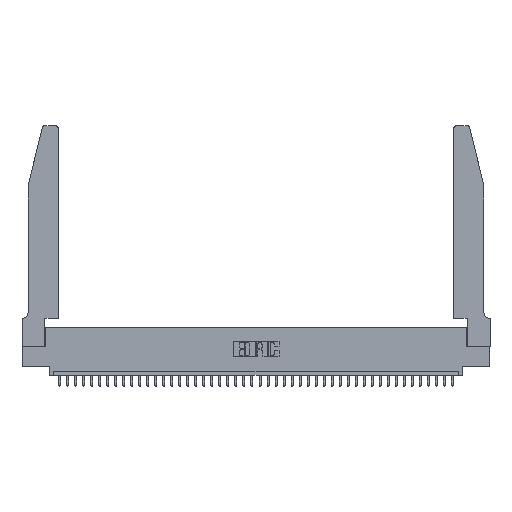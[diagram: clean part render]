
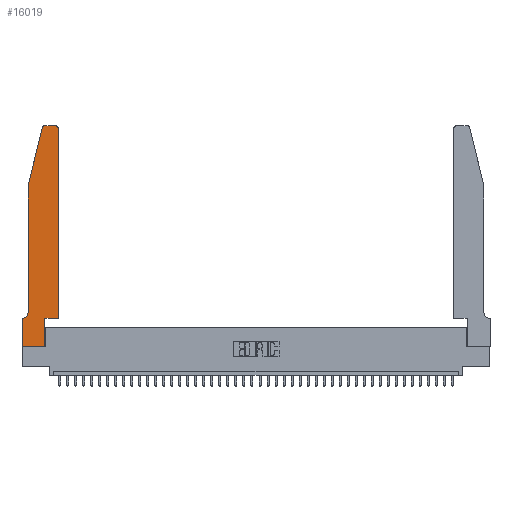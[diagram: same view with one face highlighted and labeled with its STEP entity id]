
A CAD part, top view. The second image highlights one B-rep face of the part: STEP entity #16019.
In plain terms, the highlighted planar face has unit normal (0, 0, 1).
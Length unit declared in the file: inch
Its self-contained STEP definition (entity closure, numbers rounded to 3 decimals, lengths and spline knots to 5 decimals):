
#346 = CARTESIAN_POINT ( 'NONE',  ( 0.25487, 2.72718, 0.37 ) ) ;
#736 = DIRECTION ( 'NONE',  ( -1., 0., 0. ) ) ;
#814 = EDGE_CURVE ( 'NONE', #9112, #20167, #5189, .T. ) ;
#1764 = AXIS2_PLACEMENT_3D ( 'NONE', #19782, #19914, #736 ) ;
#2838 = CARTESIAN_POINT ( 'NONE',  ( 0.4505, 0.35, 0.37 ) ) ;
#3013 = VERTEX_POINT ( 'NONE', #36718 ) ;
#3801 = ORIENTED_EDGE ( 'NONE', *, *, #39092, .T. ) ;
#3964 = ORIENTED_EDGE ( 'NONE', *, *, #16819, .T. ) ;
#4105 = CARTESIAN_POINT ( 'NONE',  ( 0., 0., 0.37 ) ) ;
#4216 = DIRECTION ( 'NONE',  ( 0., 1., 0. ) ) ;
#4330 = CARTESIAN_POINT ( 'NONE',  ( 0.4505, 0.35, 0.37 ) ) ;
#5189 = LINE ( 'NONE', #28190, #39154 ) ;
#5357 = DIRECTION ( 'NONE',  ( 1., 0., 0. ) ) ;
#5396 = VECTOR ( 'NONE', #35546, 39.37008 ) ;
#6058 = VERTEX_POINT ( 'NONE', #20160 ) ;
#6128 = ORIENTED_EDGE ( 'NONE', *, *, #37053, .T. ) ;
#6854 = ORIENTED_EDGE ( 'NONE', *, *, #814, .T. ) ;
#7038 = ORIENTED_EDGE ( 'NONE', *, *, #9373, .T. ) ;
#7457 = LINE ( 'NONE', #18163, #25952 ) ;
#8942 = LINE ( 'NONE', #23212, #30993 ) ;
#9038 = ORIENTED_EDGE ( 'NONE', *, *, #20512, .T. ) ;
#9095 = ORIENTED_EDGE ( 'NONE', *, *, #15731, .T. ) ;
#9112 = VERTEX_POINT ( 'NONE', #40099 ) ;
#9202 = CARTESIAN_POINT ( 'NONE',  ( 0., 0., 0.37 ) ) ;
#9373 = EDGE_CURVE ( 'NONE', #20611, #40476, #41179, .T. ) ;
#9575 = CARTESIAN_POINT ( 'NONE',  ( 0.0755, 0.35, 0.37 ) ) ;
#10657 = CARTESIAN_POINT ( 'NONE',  ( 0.4505, 0.35, 0.37 ) ) ;
#10990 = VECTOR ( 'NONE', #4216, 39.37008 ) ;
#11147 = ORIENTED_EDGE ( 'NONE', *, *, #37629, .T. ) ;
#11154 = VECTOR ( 'NONE', #32223, 39.37008 ) ;
#11833 = LINE ( 'NONE', #2838, #12321 ) ;
#12281 = VECTOR ( 'NONE', #18586, 39.37008 ) ;
#12321 = VECTOR ( 'NONE', #25205, 39.37008 ) ;
#12413 = DIRECTION ( 'NONE',  ( 1., 0., 0. ) ) ;
#12538 = AXIS2_PLACEMENT_3D ( 'NONE', #27901, #40463, #5357 ) ;
#12904 = EDGE_CURVE ( 'NONE', #3013, #34636, #13747, .T. ) ;
#13071 = VERTEX_POINT ( 'NONE', #23274 ) ;
#13747 = CIRCLE ( 'NONE', #12538, 0.03 ) ;
#14055 = EDGE_CURVE ( 'NONE', #18879, #13071, #20097, .T. ) ;
#14204 = AXIS2_PLACEMENT_3D ( 'NONE', #18815, #34764, #12413 ) ;
#15124 = CARTESIAN_POINT ( 'NONE',  ( 0.0755, 2., 0.37 ) ) ;
#15313 = DIRECTION ( 'NONE',  ( 0., -1., 0. ) ) ;
#15731 = EDGE_CURVE ( 'NONE', #34792, #18879, #19470, .T. ) ;
#16019 = ADVANCED_FACE ( 'NONE', ( #33484 ), #28220, .T. ) ;
#16699 = CARTESIAN_POINT ( 'NONE',  ( 0., 0.35, 0.37 ) ) ;
#16819 = EDGE_CURVE ( 'NONE', #38030, #6058, #7457, .T. ) ;
#16830 = LINE ( 'NONE', #9575, #5396 ) ;
#16947 = EDGE_CURVE ( 'NONE', #40476, #38030, #8942, .T. ) ;
#17538 = DIRECTION ( 'NONE',  ( 0., 0., 1. ) ) ;
#18163 = CARTESIAN_POINT ( 'NONE',  ( 0.2865, 0.35, 0.37 ) ) ;
#18586 = DIRECTION ( 'NONE',  ( -1., 0., 0. ) ) ;
#18645 = ORIENTED_EDGE ( 'NONE', *, *, #40239, .T. ) ;
#18815 = CARTESIAN_POINT ( 'NONE',  ( 0., 0.35, 0.37 ) ) ;
#18879 = VERTEX_POINT ( 'NONE', #24555 ) ;
#19244 = VECTOR ( 'NONE', #24999, 39.37008 ) ;
#19470 = LINE ( 'NONE', #10657, #10990 ) ;
#19782 = CARTESIAN_POINT ( 'NONE',  ( 0.0055, 0.42, 0.37 ) ) ;
#19914 = DIRECTION ( 'NONE',  ( 0., 0., -1. ) ) ;
#20031 = CIRCLE ( 'NONE', #1764, 0.07 ) ;
#20097 = CIRCLE ( 'NONE', #22172, 0.03 ) ;
#20160 = CARTESIAN_POINT ( 'NONE',  ( 0.2865, 0.35, 0.37 ) ) ;
#20167 = VERTEX_POINT ( 'NONE', #39733 ) ;
#20512 = EDGE_CURVE ( 'NONE', #20167, #35599, #20031, .T. ) ;
#20574 = ORIENTED_EDGE ( 'NONE', *, *, #12904, .T. ) ;
#20611 = VERTEX_POINT ( 'NONE', #16699 ) ;
#20612 = CARTESIAN_POINT ( 'NONE',  ( 0.2865, 0., 0.37 ) ) ;
#22172 = AXIS2_PLACEMENT_3D ( 'NONE', #36723, #17538, #39930 ) ;
#23212 = CARTESIAN_POINT ( 'NONE',  ( 0., 0., 0.37 ) ) ;
#23274 = CARTESIAN_POINT ( 'NONE',  ( 0.4205, 2.75, 0.37 ) ) ;
#23425 = CARTESIAN_POINT ( 'NONE',  ( 0.0055, 0.35, 0.37 ) ) ;
#24555 = CARTESIAN_POINT ( 'NONE',  ( 0.4505, 2.72, 0.37 ) ) ;
#24999 = DIRECTION ( 'NONE',  ( -0.239, -0.971, 0. ) ) ;
#25205 = DIRECTION ( 'NONE',  ( 1., 0., 0. ) ) ;
#25952 = VECTOR ( 'NONE', #37494, 39.37008 ) ;
#27901 = CARTESIAN_POINT ( 'NONE',  ( 0.284, 2.72, 0.37 ) ) ;
#28190 = CARTESIAN_POINT ( 'NONE',  ( 0.0755, 2., 0.37 ) ) ;
#28220 = PLANE ( 'NONE',  #14204 ) ;
#28769 = LINE ( 'NONE', #40569, #12281 ) ;
#30993 = VECTOR ( 'NONE', #33048, 39.37008 ) ;
#32223 = DIRECTION ( 'NONE',  ( 0., -1., 0. ) ) ;
#33048 = DIRECTION ( 'NONE',  ( 1., 0., 0. ) ) ;
#33484 = FACE_OUTER_BOUND ( 'NONE', #38317, .T. ) ;
#33564 = ORIENTED_EDGE ( 'NONE', *, *, #16947, .T. ) ;
#34273 = ORIENTED_EDGE ( 'NONE', *, *, #14055, .T. ) ;
#34636 = VERTEX_POINT ( 'NONE', #346 ) ;
#34764 = DIRECTION ( 'NONE',  ( 0., 0., 1. ) ) ;
#34792 = VERTEX_POINT ( 'NONE', #4330 ) ;
#35546 = DIRECTION ( 'NONE',  ( -1., 0., 0. ) ) ;
#35599 = VERTEX_POINT ( 'NONE', #23425 ) ;
#36718 = CARTESIAN_POINT ( 'NONE',  ( 0.284, 2.75, 0.37 ) ) ;
#36723 = CARTESIAN_POINT ( 'NONE',  ( 0.4205, 2.72, 0.37 ) ) ;
#37053 = EDGE_CURVE ( 'NONE', #6058, #34792, #11833, .T. ) ;
#37494 = DIRECTION ( 'NONE',  ( 0., 1., 0. ) ) ;
#37629 = EDGE_CURVE ( 'NONE', #13071, #3013, #28769, .T. ) ;
#38030 = VERTEX_POINT ( 'NONE', #20612 ) ;
#38317 = EDGE_LOOP ( 'NONE', ( #11147, #20574, #18645, #6854, #9038, #3801, #7038, #33564, #3964, #6128, #9095, #34273 ) ) ;
#39092 = EDGE_CURVE ( 'NONE', #35599, #20611, #16830, .T. ) ;
#39154 = VECTOR ( 'NONE', #15313, 39.37008 ) ;
#39237 = LINE ( 'NONE', #15124, #19244 ) ;
#39733 = CARTESIAN_POINT ( 'NONE',  ( 0.0755, 0.42, 0.37 ) ) ;
#39930 = DIRECTION ( 'NONE',  ( 1., 0., 0. ) ) ;
#40099 = CARTESIAN_POINT ( 'NONE',  ( 0.0755, 2., 0.37 ) ) ;
#40239 = EDGE_CURVE ( 'NONE', #34636, #9112, #39237, .T. ) ;
#40463 = DIRECTION ( 'NONE',  ( 0., 0., 1. ) ) ;
#40476 = VERTEX_POINT ( 'NONE', #4105 ) ;
#40569 = CARTESIAN_POINT ( 'NONE',  ( 0.2605, 2.75, 0.37 ) ) ;
#41179 = LINE ( 'NONE', #9202, #11154 ) ;
